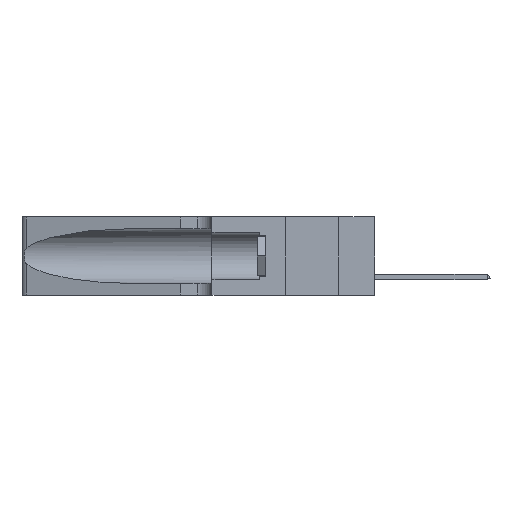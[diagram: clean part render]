
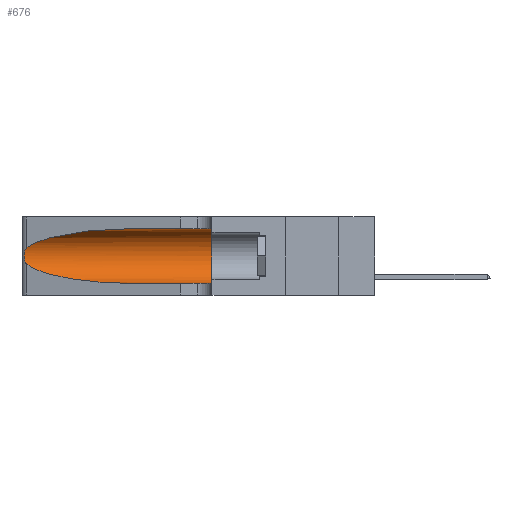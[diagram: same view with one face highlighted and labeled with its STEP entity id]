
A CAD part, left-side view. The second image highlights one B-rep face of the part: STEP entity #676.
In plain terms, the highlighted cylindrical face has radius 3.308 mm (diameter 6.617 mm), a partial arc.
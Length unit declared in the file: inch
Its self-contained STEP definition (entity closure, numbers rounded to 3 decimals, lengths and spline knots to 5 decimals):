
#676 = ADVANCED_FACE ( 'NONE', ( #1975 ), #5302, .F. ) ;
#865 = CARTESIAN_POINT ( 'NONE',  ( 0.1305, 0.72297, 0.31525 ) ) ;
#1287 = CARTESIAN_POINT ( 'NONE',  ( 0.25856, 1.23593, 0.16098 ) ) ;
#1975 = FACE_OUTER_BOUND ( 'NONE', #23861, .T. ) ;
#2623 = VECTOR ( 'NONE', #8032, 39.37008 ) ;
#3653 = AXIS2_PLACEMENT_3D ( 'NONE', #24898, #14403, #39116 ) ;
#4008 = AXIS2_PLACEMENT_3D ( 'NONE', #25175, #14854, #17943 ) ;
#4226 = CARTESIAN_POINT ( 'NONE',  ( 0.1305, 0.72297, 0.31525 ) ) ;
#4694 = CARTESIAN_POINT ( 'NONE',  ( 0.25555, 1.22994, 0.2215 ) ) ;
#4702 = VERTEX_POINT ( 'NONE', #40809 ) ;
#5302 = CYLINDRICAL_SURFACE ( 'NONE', #4008, 0.13025 ) ;
#7912 = CARTESIAN_POINT ( 'NONE',  ( 0.2373, 1.15595, 0.28018 ) ) ;
#8032 = DIRECTION ( 'NONE',  ( 0., -1., 0. ) ) ;
#10032 = CARTESIAN_POINT ( 'NONE',  ( 0.25487, 1.22718, 0.14631 ) ) ;
#10183 = ORIENTED_EDGE ( 'NONE', *, *, #28312, .T. ) ;
#10882 = EDGE_CURVE ( 'NONE', #11871, #40105, #22432, .T. ) ;
#11524 = ORIENTED_EDGE ( 'NONE', *, *, #22505, .T. ) ;
#11871 = VERTEX_POINT ( 'NONE', #865 ) ;
#11889 = CARTESIAN_POINT ( 'NONE',  ( 0.26075, 1.23896, 0.178 ) ) ;
#12897 =( BOUNDED_CURVE ( )  B_SPLINE_CURVE ( 3, ( #4226, #21745, #7912, #18220 ),
 .UNSPECIFIED., .F., .T. ) 
 B_SPLINE_CURVE_WITH_KNOTS ( ( 4, 4 ),
 ( 1.5708, 2.84003 ),
 .UNSPECIFIED. ) 
 CURVE ( )  GEOMETRIC_REPRESENTATION_ITEM ( )  RATIONAL_B_SPLINE_CURVE ( ( 1., 0.87, 0.87, 1. ) ) 
 REPRESENTATION_ITEM ( '' )  );
#14403 = DIRECTION ( 'NONE',  ( 0., 1., 0. ) ) ;
#14854 = DIRECTION ( 'NONE',  ( 0., -1., 0. ) ) ;
#14985 = VERTEX_POINT ( 'NONE', #10032 ) ;
#14990 = CARTESIAN_POINT ( 'NONE',  ( 0.26017, 1.23833, 0.17102 ) ) ;
#15465 = CARTESIAN_POINT ( 'NONE',  ( 0.25555, 1.22993, 0.14849 ) ) ;
#16340 = ORIENTED_EDGE ( 'NONE', *, *, #10882, .F. ) ;
#16521 = ORIENTED_EDGE ( 'NONE', *, *, #43806, .T. ) ;
#17661 =( BOUNDED_CURVE ( )  B_SPLINE_CURVE ( 3, ( #30523, #31109, #20302, #45162 ),
 .UNSPECIFIED., .F., .T. ) 
 B_SPLINE_CURVE_WITH_KNOTS ( ( 4, 4 ),
 ( 3.44316, 4.71239 ),
 .UNSPECIFIED. ) 
 CURVE ( )  GEOMETRIC_REPRESENTATION_ITEM ( )  RATIONAL_B_SPLINE_CURVE ( ( 1., 0.87, 0.87, 1. ) ) 
 REPRESENTATION_ITEM ( '' )  );
#17943 = DIRECTION ( 'NONE',  ( 0., 0., -1. ) ) ;
#18220 = CARTESIAN_POINT ( 'NONE',  ( 0.25487, 1.22718, 0.22369 ) ) ;
#19147 = CARTESIAN_POINT ( 'NONE',  ( 0.25487, 1.22718, 0.14631 ) ) ;
#19811 = CARTESIAN_POINT ( 'NONE',  ( 0.25487, 1.22718, 0.22369 ) ) ;
#20302 = CARTESIAN_POINT ( 'NONE',  ( 0.18966, 0.96281, 0.05475 ) ) ;
#20336 = ORIENTED_EDGE ( 'NONE', *, *, #39027, .T. ) ;
#21043 = B_SPLINE_CURVE_WITH_KNOTS ( 'NONE', 3,
 ( #36486, #4694, #39995, #25621, #22395, #36155, #22708, #11889, #14990, #1287, #25952, #36640, #15465, #19147 ),
 .UNSPECIFIED., .F., .F.,
 ( 4, 2, 2, 2, 2, 2, 4 ),
 ( 0., 0.00027, 0.00053, 0.00107, 0.0016, 0.00187, 0.00214 ),
 .UNSPECIFIED. ) ;
#21116 = VERTEX_POINT ( 'NONE', #33440 ) ;
#21745 = CARTESIAN_POINT ( 'NONE',  ( 0.18966, 0.96281, 0.31525 ) ) ;
#22395 = CARTESIAN_POINT ( 'NONE',  ( 0.25854, 1.2359, 0.20912 ) ) ;
#22432 = LINE ( 'NONE', #22507, #2623 ) ;
#22505 = EDGE_CURVE ( 'NONE', #11871, #43732, #12897, .T. ) ;
#22507 = CARTESIAN_POINT ( 'NONE',  ( 0.1305, 1.61858, 0.31525 ) ) ;
#22708 = CARTESIAN_POINT ( 'NONE',  ( 0.26075, 1.23896, 0.19203 ) ) ;
#23472 = CARTESIAN_POINT ( 'NONE',  ( 0.1305, 0.35, 0.31525 ) ) ;
#23861 = EDGE_LOOP ( 'NONE', ( #11524, #10183, #20336, #16521, #38827, #16340 ) ) ;
#24898 = CARTESIAN_POINT ( 'NONE',  ( 0.1305, 0.35, 0.185 ) ) ;
#25175 = CARTESIAN_POINT ( 'NONE',  ( 0.1305, 1.61858, 0.185 ) ) ;
#25621 = CARTESIAN_POINT ( 'NONE',  ( 0.25787, 1.23484, 0.2124 ) ) ;
#25952 = CARTESIAN_POINT ( 'NONE',  ( 0.25789, 1.23486, 0.15765 ) ) ;
#28003 = CARTESIAN_POINT ( 'NONE',  ( 0.1305, 1.61858, 0.05475 ) ) ;
#28312 = EDGE_CURVE ( 'NONE', #43732, #14985, #21043, .T. ) ;
#30395 = EDGE_CURVE ( 'NONE', #40105, #4702, #43577, .T. ) ;
#30523 = CARTESIAN_POINT ( 'NONE',  ( 0.25487, 1.22718, 0.14631 ) ) ;
#31109 = CARTESIAN_POINT ( 'NONE',  ( 0.2373, 1.15595, 0.08982 ) ) ;
#33440 = CARTESIAN_POINT ( 'NONE',  ( 0.1305, 0.72297, 0.05475 ) ) ;
#36155 = CARTESIAN_POINT ( 'NONE',  ( 0.26018, 1.23835, 0.19895 ) ) ;
#36486 = CARTESIAN_POINT ( 'NONE',  ( 0.25487, 1.22718, 0.22369 ) ) ;
#36640 = CARTESIAN_POINT ( 'NONE',  ( 0.25639, 1.23186, 0.15144 ) ) ;
#38827 = ORIENTED_EDGE ( 'NONE', *, *, #30395, .F. ) ;
#39027 = EDGE_CURVE ( 'NONE', #14985, #21116, #17661, .T. ) ;
#39116 = DIRECTION ( 'NONE',  ( 0., 0., 1. ) ) ;
#39995 = CARTESIAN_POINT ( 'NONE',  ( 0.25639, 1.23184, 0.21858 ) ) ;
#40105 = VERTEX_POINT ( 'NONE', #23472 ) ;
#40535 = VECTOR ( 'NONE', #42182, 39.37008 ) ;
#40809 = CARTESIAN_POINT ( 'NONE',  ( 0.1305, 0.35, 0.05475 ) ) ;
#42182 = DIRECTION ( 'NONE',  ( 0., -1., 0. ) ) ;
#42708 = LINE ( 'NONE', #28003, #40535 ) ;
#43577 = CIRCLE ( 'NONE', #3653, 0.13025 ) ;
#43732 = VERTEX_POINT ( 'NONE', #19811 ) ;
#43806 = EDGE_CURVE ( 'NONE', #21116, #4702, #42708, .T. ) ;
#45162 = CARTESIAN_POINT ( 'NONE',  ( 0.1305, 0.72297, 0.05475 ) ) ;
